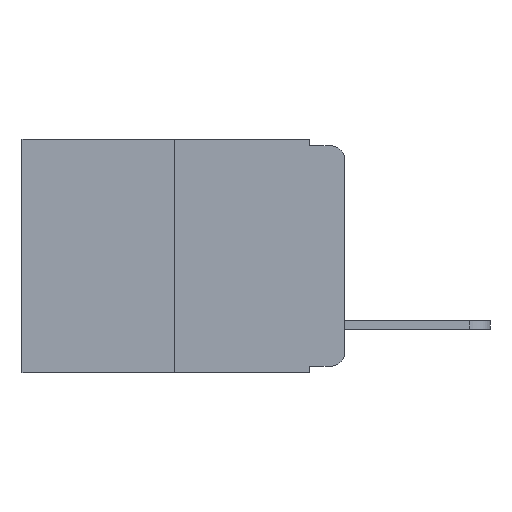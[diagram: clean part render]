
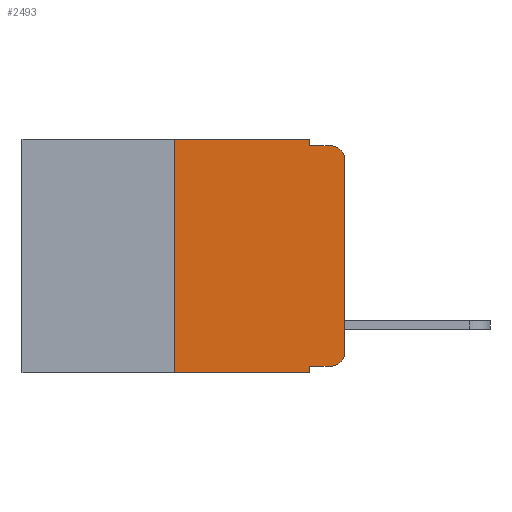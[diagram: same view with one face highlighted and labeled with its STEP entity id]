
A CAD part, left-side view. The second image highlights one B-rep face of the part: STEP entity #2493.
In plain terms, the highlighted planar face has unit normal (-1, 0, 0).
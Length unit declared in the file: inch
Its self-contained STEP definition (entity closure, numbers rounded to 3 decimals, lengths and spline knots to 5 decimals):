
#188 = ORIENTED_EDGE ( 'NONE', *, *, #3706, .T. ) ;
#323 = DIRECTION ( 'NONE',  ( 1., 0., 0. ) ) ;
#411 = CARTESIAN_POINT ( 'NONE',  ( 0., 0.051, -0.01 ) ) ;
#576 = CARTESIAN_POINT ( 'NONE',  ( 0., 0.25, -0.343 ) ) ;
#703 = EDGE_CURVE ( 'NONE', #5487, #18246, #9946, .T. ) ;
#816 = DIRECTION ( 'NONE',  ( 0., -1., 0. ) ) ;
#941 = CARTESIAN_POINT ( 'NONE',  ( 0., 0.02, -0.03 ) ) ;
#990 = LINE ( 'NONE', #5650, #20134 ) ;
#1426 = VECTOR ( 'NONE', #14471, 39.37008 ) ;
#2110 = CARTESIAN_POINT ( 'NONE',  ( 0., 0.051, 0. ) ) ;
#2301 = ORIENTED_EDGE ( 'NONE', *, *, #7297, .F. ) ;
#2351 = CARTESIAN_POINT ( 'NONE',  ( 0., 0.051, -0.343 ) ) ;
#2415 = VERTEX_POINT ( 'NONE', #8597 ) ;
#2493 = ADVANCED_FACE ( 'NONE', ( #16758 ), #15608, .F. ) ;
#2845 = CARTESIAN_POINT ( 'NONE',  ( 0., 0., 0. ) ) ;
#3191 = DIRECTION ( 'NONE',  ( 0., 0., -1. ) ) ;
#3249 = DIRECTION ( 'NONE',  ( 0., 0., -1. ) ) ;
#3660 = DIRECTION ( 'NONE',  ( 0., -1., 0. ) ) ;
#3706 = EDGE_CURVE ( 'NONE', #18246, #4266, #12236, .T. ) ;
#3812 = VECTOR ( 'NONE', #816, 39.37008 ) ;
#4266 = VERTEX_POINT ( 'NONE', #9828 ) ;
#4700 = ORIENTED_EDGE ( 'NONE', *, *, #20724, .F. ) ;
#4704 = CIRCLE ( 'NONE', #18248, 0.02 ) ;
#4938 = AXIS2_PLACEMENT_3D ( 'NONE', #15576, #20946, #22361 ) ;
#5354 = ORIENTED_EDGE ( 'NONE', *, *, #23116, .T. ) ;
#5431 = CARTESIAN_POINT ( 'NONE',  ( 0., 0.473, 0. ) ) ;
#5487 = VERTEX_POINT ( 'NONE', #17976 ) ;
#5650 = CARTESIAN_POINT ( 'NONE',  ( 0., 0.25, 0. ) ) ;
#5855 = AXIS2_PLACEMENT_3D ( 'NONE', #5431, #323, #3191 ) ;
#6321 = EDGE_CURVE ( 'NONE', #15274, #5487, #23137, .T. ) ;
#6781 = EDGE_CURVE ( 'NONE', #16048, #18405, #8749, .T. ) ;
#7297 = EDGE_CURVE ( 'NONE', #18405, #9847, #18304, .T. ) ;
#7988 = DIRECTION ( 'NONE',  ( 0., 0., -1. ) ) ;
#8366 = CARTESIAN_POINT ( 'NONE',  ( 0., 0.02, -0.01 ) ) ;
#8394 = ORIENTED_EDGE ( 'NONE', *, *, #6781, .F. ) ;
#8417 = ORIENTED_EDGE ( 'NONE', *, *, #6321, .T. ) ;
#8597 = CARTESIAN_POINT ( 'NONE',  ( 0., 0.25, 0. ) ) ;
#8749 = LINE ( 'NONE', #2110, #23117 ) ;
#9117 = LINE ( 'NONE', #22267, #3812 ) ;
#9828 = CARTESIAN_POINT ( 'NONE',  ( 0., 0., -0.03 ) ) ;
#9847 = VERTEX_POINT ( 'NONE', #8366 ) ;
#9946 = CIRCLE ( 'NONE', #4938, 0.02 ) ;
#10220 = EDGE_CURVE ( 'NONE', #15274, #12750, #11510, .T. ) ;
#10646 = VECTOR ( 'NONE', #24543, 39.37008 ) ;
#11510 = LINE ( 'NONE', #22459, #12148 ) ;
#12148 = VECTOR ( 'NONE', #22410, 39.37008 ) ;
#12236 = LINE ( 'NONE', #2845, #1426 ) ;
#12750 = VERTEX_POINT ( 'NONE', #2351 ) ;
#13015 = EDGE_LOOP ( 'NONE', ( #188, #21728, #2301, #8394, #14795, #4700, #5354, #21752, #8417, #13612 ) ) ;
#13045 = CARTESIAN_POINT ( 'NONE',  ( 0., 0.051, -0.333 ) ) ;
#13612 = ORIENTED_EDGE ( 'NONE', *, *, #703, .T. ) ;
#13961 = VECTOR ( 'NONE', #16163, 39.37008 ) ;
#14471 = DIRECTION ( 'NONE',  ( 0., 0., 1. ) ) ;
#14795 = ORIENTED_EDGE ( 'NONE', *, *, #22825, .F. ) ;
#15051 = DIRECTION ( 'NONE',  ( -1., 0., 0. ) ) ;
#15213 = VERTEX_POINT ( 'NONE', #576 ) ;
#15274 = VERTEX_POINT ( 'NONE', #13045 ) ;
#15468 = CARTESIAN_POINT ( 'NONE',  ( 0., 0.051, -0.333 ) ) ;
#15576 = CARTESIAN_POINT ( 'NONE',  ( 0., 0.02, -0.313 ) ) ;
#15608 = PLANE ( 'NONE',  #5855 ) ;
#15774 = LINE ( 'NONE', #19214, #10646 ) ;
#16048 = VERTEX_POINT ( 'NONE', #21285 ) ;
#16060 = CARTESIAN_POINT ( 'NONE',  ( 0., 0.051, -0.01 ) ) ;
#16163 = DIRECTION ( 'NONE',  ( 0., -1., 0. ) ) ;
#16758 = FACE_OUTER_BOUND ( 'NONE', #13015, .T. ) ;
#17749 = VECTOR ( 'NONE', #3660, 39.37008 ) ;
#17976 = CARTESIAN_POINT ( 'NONE',  ( 0., 0.02, -0.333 ) ) ;
#18246 = VERTEX_POINT ( 'NONE', #23302 ) ;
#18248 = AXIS2_PLACEMENT_3D ( 'NONE', #941, #15051, #3249 ) ;
#18304 = LINE ( 'NONE', #16060, #17749 ) ;
#18405 = VERTEX_POINT ( 'NONE', #411 ) ;
#19214 = CARTESIAN_POINT ( 'NONE',  ( 0., 0.473, 0. ) ) ;
#20134 = VECTOR ( 'NONE', #22692, 39.37008 ) ;
#20724 = EDGE_CURVE ( 'NONE', #15213, #2415, #990, .T. ) ;
#20946 = DIRECTION ( 'NONE',  ( -1., 0., 0. ) ) ;
#21285 = CARTESIAN_POINT ( 'NONE',  ( 0., 0.051, 0. ) ) ;
#21728 = ORIENTED_EDGE ( 'NONE', *, *, #24484, .T. ) ;
#21752 = ORIENTED_EDGE ( 'NONE', *, *, #10220, .F. ) ;
#22267 = CARTESIAN_POINT ( 'NONE',  ( 0., 0.473, -0.343 ) ) ;
#22361 = DIRECTION ( 'NONE',  ( 0., 0., -1. ) ) ;
#22410 = DIRECTION ( 'NONE',  ( 0., 0., -1. ) ) ;
#22459 = CARTESIAN_POINT ( 'NONE',  ( 0., 0.051, 0. ) ) ;
#22692 = DIRECTION ( 'NONE',  ( 0., 0., 1. ) ) ;
#22825 = EDGE_CURVE ( 'NONE', #2415, #16048, #15774, .T. ) ;
#23116 = EDGE_CURVE ( 'NONE', #15213, #12750, #9117, .T. ) ;
#23117 = VECTOR ( 'NONE', #7988, 39.37008 ) ;
#23137 = LINE ( 'NONE', #15468, #13961 ) ;
#23302 = CARTESIAN_POINT ( 'NONE',  ( 0., 0., -0.313 ) ) ;
#24484 = EDGE_CURVE ( 'NONE', #4266, #9847, #4704, .T. ) ;
#24543 = DIRECTION ( 'NONE',  ( 0., -1., 0. ) ) ;
